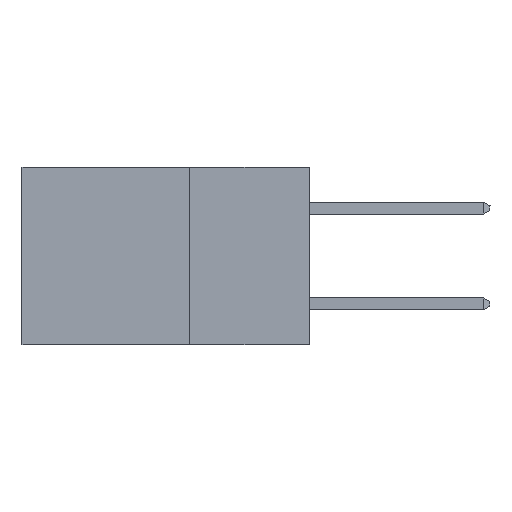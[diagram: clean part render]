
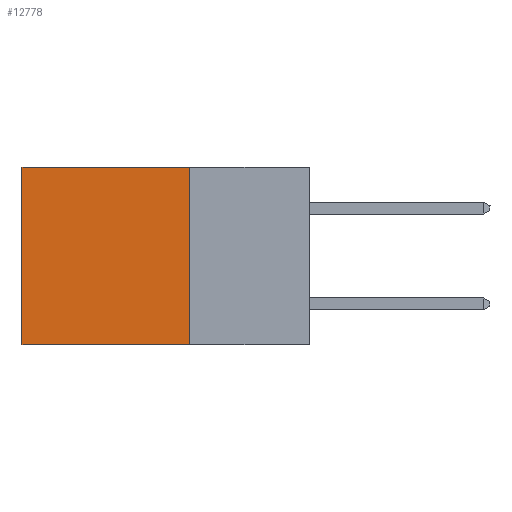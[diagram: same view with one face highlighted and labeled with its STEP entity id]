
A CAD part, left-side view. The second image highlights one B-rep face of the part: STEP entity #12778.
In plain terms, the highlighted planar face has unit normal (-1, 0, 0).
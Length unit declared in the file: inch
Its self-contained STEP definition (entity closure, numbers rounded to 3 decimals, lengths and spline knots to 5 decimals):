
#339 = CARTESIAN_POINT ( 'NONE',  ( 0.2875, 0.6, 0. ) ) ;
#812 = ORIENTED_EDGE ( 'NONE', *, *, #11902, .F. ) ;
#1894 = VERTEX_POINT ( 'NONE', #2605 ) ;
#1984 = VERTEX_POINT ( 'NONE', #18477 ) ;
#2449 = EDGE_LOOP ( 'NONE', ( #7066, #812, #12445, #17394 ) ) ;
#2521 = DIRECTION ( 'NONE',  ( 0., 0., -1. ) ) ;
#2605 = CARTESIAN_POINT ( 'NONE',  ( 0.2875, 0.25, -0.37 ) ) ;
#2957 = VECTOR ( 'NONE', #17274, 39.37008 ) ;
#5035 = AXIS2_PLACEMENT_3D ( 'NONE', #8748, #11669, #2521 ) ;
#5115 = CARTESIAN_POINT ( 'NONE',  ( 0.2875, 0.25, 0. ) ) ;
#5603 = CARTESIAN_POINT ( 'NONE',  ( 0.2875, 0.6, 0. ) ) ;
#5901 = VECTOR ( 'NONE', #16985, 39.37008 ) ;
#6174 = EDGE_CURVE ( 'NONE', #15429, #1894, #9973, .T. ) ;
#6341 = EDGE_CURVE ( 'NONE', #15429, #16909, #15374, .T. ) ;
#6604 = CARTESIAN_POINT ( 'NONE',  ( 0.2875, 0.25, 0. ) ) ;
#6677 = DIRECTION ( 'NONE',  ( 0., 0., -1. ) ) ;
#7066 = ORIENTED_EDGE ( 'NONE', *, *, #13873, .T. ) ;
#7925 = DIRECTION ( 'NONE',  ( 0., 1., 0. ) ) ;
#7962 = LINE ( 'NONE', #339, #18928 ) ;
#8748 = CARTESIAN_POINT ( 'NONE',  ( 0.2875, 0.25, 0. ) ) ;
#9973 = LINE ( 'NONE', #5115, #5901 ) ;
#10229 = PLANE ( 'NONE',  #5035 ) ;
#11574 = CARTESIAN_POINT ( 'NONE',  ( 0.2875, 0.25, 0. ) ) ;
#11669 = DIRECTION ( 'NONE',  ( 1., 0., 0. ) ) ;
#11902 = EDGE_CURVE ( 'NONE', #1894, #1984, #19232, .T. ) ;
#12445 = ORIENTED_EDGE ( 'NONE', *, *, #6174, .F. ) ;
#12778 = ADVANCED_FACE ( 'NONE', ( #15013 ), #10229, .F. ) ;
#13873 = EDGE_CURVE ( 'NONE', #16909, #1984, #7962, .T. ) ;
#15013 = FACE_OUTER_BOUND ( 'NONE', #2449, .T. ) ;
#15047 = VECTOR ( 'NONE', #7925, 39.37008 ) ;
#15154 = CARTESIAN_POINT ( 'NONE',  ( 0.2875, 0.25, -0.37 ) ) ;
#15374 = LINE ( 'NONE', #11574, #2957 ) ;
#15429 = VERTEX_POINT ( 'NONE', #6604 ) ;
#16909 = VERTEX_POINT ( 'NONE', #5603 ) ;
#16985 = DIRECTION ( 'NONE',  ( 0., 0., -1. ) ) ;
#17274 = DIRECTION ( 'NONE',  ( 0., 1., 0. ) ) ;
#17394 = ORIENTED_EDGE ( 'NONE', *, *, #6341, .T. ) ;
#18477 = CARTESIAN_POINT ( 'NONE',  ( 0.2875, 0.6, -0.37 ) ) ;
#18928 = VECTOR ( 'NONE', #6677, 39.37008 ) ;
#19232 = LINE ( 'NONE', #15154, #15047 ) ;
